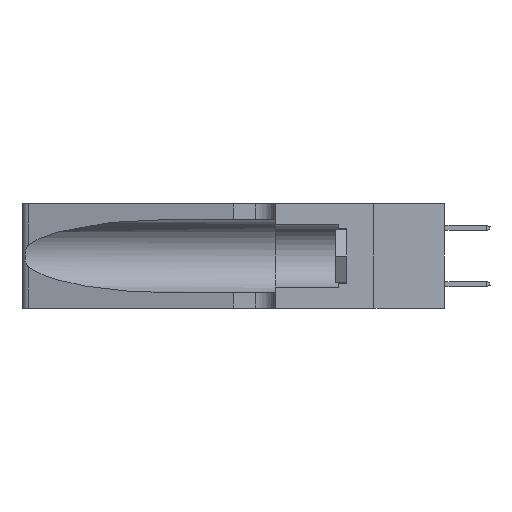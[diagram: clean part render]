
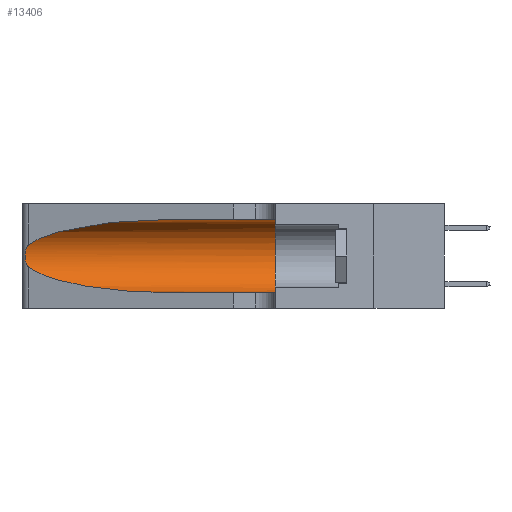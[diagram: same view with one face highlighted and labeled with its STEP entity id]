
A CAD part, left-side view. The second image highlights one B-rep face of the part: STEP entity #13406.
In plain terms, the highlighted cylindrical face has radius 3.308 mm (diameter 6.617 mm), a partial arc.
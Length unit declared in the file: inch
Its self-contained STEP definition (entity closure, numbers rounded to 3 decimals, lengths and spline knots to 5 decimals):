
#539 = CIRCLE ( 'NONE', #27518, 0.13025 ) ;
#1578 = ORIENTED_EDGE ( 'NONE', *, *, #21805, .T. ) ;
#1955 = CARTESIAN_POINT ( 'NONE',  ( 0.25639, 1.23184, 0.21858 ) ) ;
#2788 = LINE ( 'NONE', #13273, #6174 ) ;
#3599 =( BOUNDED_CURVE ( )  B_SPLINE_CURVE ( 3, ( #11092, #9001, #11467, #24312 ),
 .UNSPECIFIED., .F., .F. ) 
 B_SPLINE_CURVE_WITH_KNOTS ( ( 4, 4 ),
 ( 3.44316, 4.71239 ),
 .UNSPECIFIED. ) 
 CURVE ( )  GEOMETRIC_REPRESENTATION_ITEM ( )  RATIONAL_B_SPLINE_CURVE ( ( 1., 0.87, 0.87, 1. ) ) 
 REPRESENTATION_ITEM ( '' )  );
#4120 = CARTESIAN_POINT ( 'NONE',  ( 0.1305, 1.61858, 0.31525 ) ) ;
#4180 = VERTEX_POINT ( 'NONE', #5717 ) ;
#4263 = ORIENTED_EDGE ( 'NONE', *, *, #9295, .T. ) ;
#4413 = DIRECTION ( 'NONE',  ( 0., -1., 0. ) ) ;
#4471 = CARTESIAN_POINT ( 'NONE',  ( 0.25555, 1.22993, 0.14849 ) ) ;
#5471 = CARTESIAN_POINT ( 'NONE',  ( 0.1305, 0.35, 0.185 ) ) ;
#5717 = CARTESIAN_POINT ( 'NONE',  ( 0.1305, 0.35, 0.05475 ) ) ;
#6174 = VECTOR ( 'NONE', #4413, 39.37008 ) ;
#6917 = VERTEX_POINT ( 'NONE', #26499 ) ;
#7258 = CARTESIAN_POINT ( 'NONE',  ( 0.18966, 0.96281, 0.31525 ) ) ;
#7294 = VERTEX_POINT ( 'NONE', #12038 ) ;
#7539 = DIRECTION ( 'NONE',  ( 0., 0., -1. ) ) ;
#7776 = B_SPLINE_CURVE_WITH_KNOTS ( 'NONE', 3,
 ( #17133, #21859, #1955, #19493, #26169, #19669, #23640, #17407, #15227, #26080, #25989, #13161, #4471, #10677 ),
 .UNSPECIFIED., .F., .F.,
 ( 4, 2, 2, 2, 2, 2, 4 ),
 ( 0., 0.00027, 0.00053, 0.00107, 0.0016, 0.00187, 0.00214 ),
 .UNSPECIFIED. ) ;
#9000 = EDGE_CURVE ( 'NONE', #21208, #4180, #539, .T. ) ;
#9001 = CARTESIAN_POINT ( 'NONE',  ( 0.2373, 1.15595, 0.08982 ) ) ;
#9209 = EDGE_LOOP ( 'NONE', ( #4263, #1578, #23661, #14206, #16983, #17465 ) ) ;
#9295 = EDGE_CURVE ( 'NONE', #27504, #6917, #16648, .T. ) ;
#9458 = CARTESIAN_POINT ( 'NONE',  ( 0.2373, 1.15595, 0.28018 ) ) ;
#9604 = VERTEX_POINT ( 'NONE', #26433 ) ;
#10004 = AXIS2_PLACEMENT_3D ( 'NONE', #14271, #16469, #7539 ) ;
#10677 = CARTESIAN_POINT ( 'NONE',  ( 0.25487, 1.22718, 0.14631 ) ) ;
#11092 = CARTESIAN_POINT ( 'NONE',  ( 0.25487, 1.22718, 0.14631 ) ) ;
#11467 = CARTESIAN_POINT ( 'NONE',  ( 0.18966, 0.96281, 0.05475 ) ) ;
#12038 = CARTESIAN_POINT ( 'NONE',  ( 0.1305, 0.72297, 0.05475 ) ) ;
#12599 = DIRECTION ( 'NONE',  ( 0., -1., 0. ) ) ;
#13161 = CARTESIAN_POINT ( 'NONE',  ( 0.25639, 1.23186, 0.15144 ) ) ;
#13273 = CARTESIAN_POINT ( 'NONE',  ( 0.1305, 1.61858, 0.05475 ) ) ;
#13406 = ADVANCED_FACE ( 'NONE', ( #19630 ), #25693, .F. ) ;
#14206 = ORIENTED_EDGE ( 'NONE', *, *, #24749, .T. ) ;
#14271 = CARTESIAN_POINT ( 'NONE',  ( 0.1305, 1.61858, 0.185 ) ) ;
#15110 = CARTESIAN_POINT ( 'NONE',  ( 0.1305, 0.72297, 0.31525 ) ) ;
#15227 = CARTESIAN_POINT ( 'NONE',  ( 0.26017, 1.23833, 0.17102 ) ) ;
#16002 = EDGE_CURVE ( 'NONE', #9604, #7294, #3599, .T. ) ;
#16469 = DIRECTION ( 'NONE',  ( 0., -1., 0. ) ) ;
#16648 =( BOUNDED_CURVE ( )  B_SPLINE_CURVE ( 3, ( #24472, #7258, #9458, #22530 ),
 .UNSPECIFIED., .F., .T. ) 
 B_SPLINE_CURVE_WITH_KNOTS ( ( 4, 4 ),
 ( 1.5708, 2.84003 ),
 .UNSPECIFIED. ) 
 CURVE ( )  GEOMETRIC_REPRESENTATION_ITEM ( )  RATIONAL_B_SPLINE_CURVE ( ( 1., 0.87, 0.87, 1. ) ) 
 REPRESENTATION_ITEM ( '' )  );
#16983 = ORIENTED_EDGE ( 'NONE', *, *, #9000, .F. ) ;
#17133 = CARTESIAN_POINT ( 'NONE',  ( 0.25487, 1.22718, 0.22369 ) ) ;
#17407 = CARTESIAN_POINT ( 'NONE',  ( 0.26075, 1.23896, 0.178 ) ) ;
#17465 = ORIENTED_EDGE ( 'NONE', *, *, #25308, .F. ) ;
#19493 = CARTESIAN_POINT ( 'NONE',  ( 0.25787, 1.23484, 0.2124 ) ) ;
#19630 = FACE_OUTER_BOUND ( 'NONE', #9209, .T. ) ;
#19669 = CARTESIAN_POINT ( 'NONE',  ( 0.26018, 1.23835, 0.19895 ) ) ;
#21107 = VECTOR ( 'NONE', #12599, 39.37008 ) ;
#21208 = VERTEX_POINT ( 'NONE', #26665 ) ;
#21467 = LINE ( 'NONE', #4120, #21107 ) ;
#21805 = EDGE_CURVE ( 'NONE', #6917, #9604, #7776, .T. ) ;
#21859 = CARTESIAN_POINT ( 'NONE',  ( 0.25555, 1.22994, 0.2215 ) ) ;
#22530 = CARTESIAN_POINT ( 'NONE',  ( 0.25487, 1.22718, 0.22369 ) ) ;
#22656 = DIRECTION ( 'NONE',  ( 0., 1., 0. ) ) ;
#23640 = CARTESIAN_POINT ( 'NONE',  ( 0.26075, 1.23896, 0.19203 ) ) ;
#23661 = ORIENTED_EDGE ( 'NONE', *, *, #16002, .T. ) ;
#24312 = CARTESIAN_POINT ( 'NONE',  ( 0.1305, 0.72297, 0.05475 ) ) ;
#24472 = CARTESIAN_POINT ( 'NONE',  ( 0.1305, 0.72297, 0.31525 ) ) ;
#24749 = EDGE_CURVE ( 'NONE', #7294, #4180, #2788, .T. ) ;
#24795 = DIRECTION ( 'NONE',  ( 0., 0., 1. ) ) ;
#25308 = EDGE_CURVE ( 'NONE', #27504, #21208, #21467, .T. ) ;
#25693 = CYLINDRICAL_SURFACE ( 'NONE', #10004, 0.13025 ) ;
#25989 = CARTESIAN_POINT ( 'NONE',  ( 0.25789, 1.23486, 0.15765 ) ) ;
#26080 = CARTESIAN_POINT ( 'NONE',  ( 0.25856, 1.23593, 0.16098 ) ) ;
#26169 = CARTESIAN_POINT ( 'NONE',  ( 0.25854, 1.2359, 0.20912 ) ) ;
#26433 = CARTESIAN_POINT ( 'NONE',  ( 0.25487, 1.22718, 0.14631 ) ) ;
#26499 = CARTESIAN_POINT ( 'NONE',  ( 0.25487, 1.22718, 0.22369 ) ) ;
#26665 = CARTESIAN_POINT ( 'NONE',  ( 0.1305, 0.35, 0.31525 ) ) ;
#27504 = VERTEX_POINT ( 'NONE', #15110 ) ;
#27518 = AXIS2_PLACEMENT_3D ( 'NONE', #5471, #22656, #24795 ) ;
